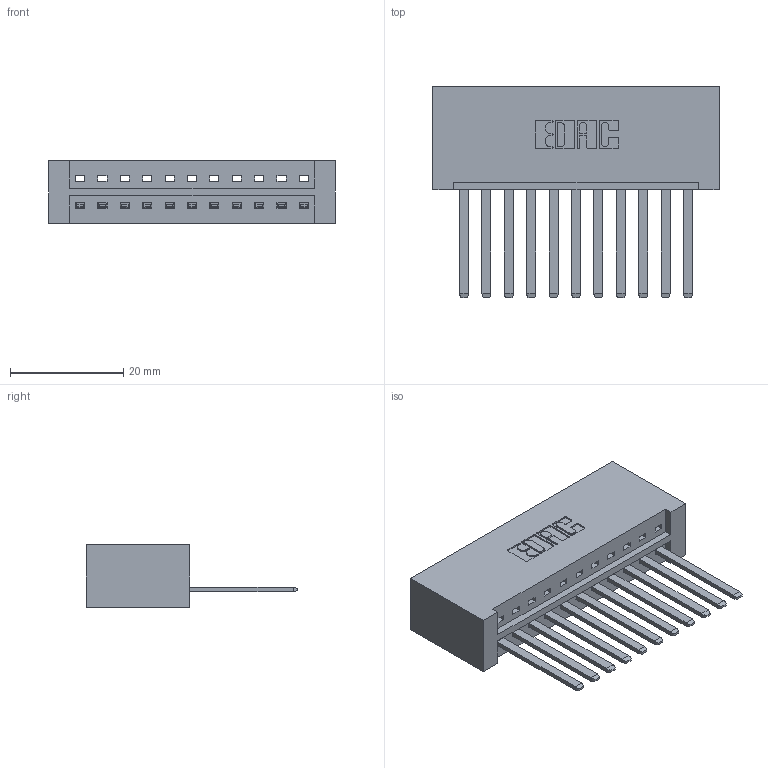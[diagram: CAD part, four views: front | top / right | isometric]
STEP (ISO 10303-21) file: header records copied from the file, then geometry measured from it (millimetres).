
FILE_DESCRIPTION (( 'STEP AP203' ), '1' );
FILE_NAME ('336-011-541-601.STEP', '2020-08-07T19:33:17', ( '' ), ( '' ), 'SwSTEP 2.0', 'SolidWorks 2020', '' );
FILE_SCHEMA (( 'CONFIG_CONTROL_DESIGN' ));
Length unit declared in the file: inch
Products named in the file (3): 336-290-001_336-290-541; 336-011-541-601; 336 Part_Lugless
Assembly tree (12 placements, depth 2):
  336-011-541-601
    336 Part_Lugless
    336-290-001_336-290-541  x11
Bounding box: 50.7 x 37.34 x 11.1 mm (x, y, z)
Volume: 8026.8 mm3; surface area: 8375 mm2
Topology: 12 solids, 12 shells, 656 faces, 1981 edges, 1312 vertices
Faces by surface type: plane 440, cylinder 216
Entity records: 11628 total; most frequent: CARTESIAN_POINT 2114, ORIENTED_EDGE 1962, DIRECTION 1739, EDGE_CURVE 981, VECTOR 857, LINE 857, VERTEX_POINT 652, AXIS2_PLACEMENT_3D 441
